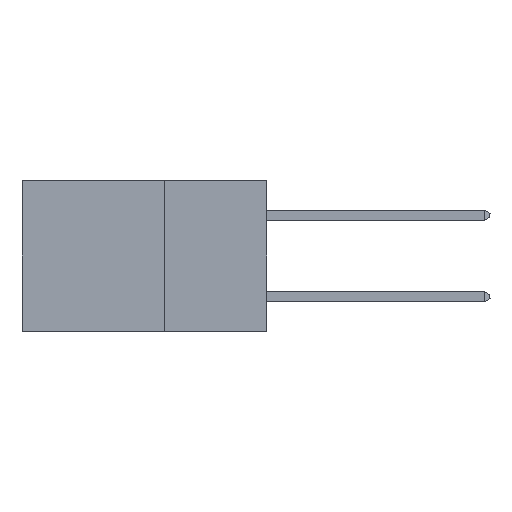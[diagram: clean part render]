
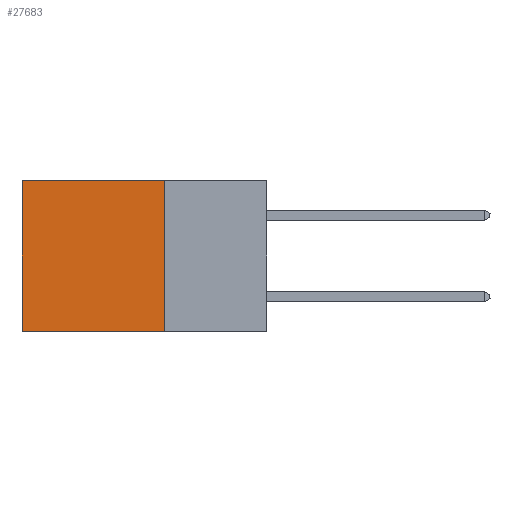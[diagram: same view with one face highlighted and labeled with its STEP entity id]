
A CAD part, left-side view. The second image highlights one B-rep face of the part: STEP entity #27683.
In plain terms, the highlighted planar face has unit normal (-1, 0, 0).
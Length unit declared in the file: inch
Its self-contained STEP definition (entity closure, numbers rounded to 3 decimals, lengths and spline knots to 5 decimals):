
#198 = ORIENTED_EDGE ( 'NONE', *, *, #32950, .F. ) ;
#1918 = CARTESIAN_POINT ( 'NONE',  ( 0.2875, 0.25, 0. ) ) ;
#1966 = EDGE_CURVE ( 'NONE', #16338, #22198, #33736, .T. ) ;
#5202 = AXIS2_PLACEMENT_3D ( 'NONE', #1918, #29483, #35114 ) ;
#5299 = EDGE_LOOP ( 'NONE', ( #31467, #198, #10802, #31281 ) ) ;
#10364 = CARTESIAN_POINT ( 'NONE',  ( 0.2875, 0.25, -0.37 ) ) ;
#10802 = ORIENTED_EDGE ( 'NONE', *, *, #34431, .F. ) ;
#13777 = VERTEX_POINT ( 'NONE', #35957 ) ;
#14352 = CARTESIAN_POINT ( 'NONE',  ( 0.2875, 0.25, 0. ) ) ;
#15483 = VECTOR ( 'NONE', #22196, 39.37008 ) ;
#16338 = VERTEX_POINT ( 'NONE', #34121 ) ;
#17976 = VECTOR ( 'NONE', #29863, 39.37008 ) ;
#19088 = VECTOR ( 'NONE', #32189, 39.37008 ) ;
#19768 = CARTESIAN_POINT ( 'NONE',  ( 0.2875, 0.25, -0.37 ) ) ;
#21308 = VERTEX_POINT ( 'NONE', #19768 ) ;
#21587 = VECTOR ( 'NONE', #33674, 39.37008 ) ;
#22196 = DIRECTION ( 'NONE',  ( 0., 0., -1. ) ) ;
#22198 = VERTEX_POINT ( 'NONE', #22245 ) ;
#22245 = CARTESIAN_POINT ( 'NONE',  ( 0.2875, 0.6, 0. ) ) ;
#22424 = LINE ( 'NONE', #30030, #15483 ) ;
#24116 = PLANE ( 'NONE',  #5202 ) ;
#24154 = EDGE_CURVE ( 'NONE', #22198, #13777, #22424, .T. ) ;
#25229 = LINE ( 'NONE', #10364, #19088 ) ;
#27683 = ADVANCED_FACE ( 'NONE', ( #29589 ), #24116, .F. ) ;
#29025 = LINE ( 'NONE', #14352, #21587 ) ;
#29483 = DIRECTION ( 'NONE',  ( 1., 0., 0. ) ) ;
#29589 = FACE_OUTER_BOUND ( 'NONE', #5299, .T. ) ;
#29863 = DIRECTION ( 'NONE',  ( 0., 1., 0. ) ) ;
#30030 = CARTESIAN_POINT ( 'NONE',  ( 0.2875, 0.6, 0. ) ) ;
#31281 = ORIENTED_EDGE ( 'NONE', *, *, #1966, .T. ) ;
#31467 = ORIENTED_EDGE ( 'NONE', *, *, #24154, .T. ) ;
#32189 = DIRECTION ( 'NONE',  ( 0., 1., 0. ) ) ;
#32950 = EDGE_CURVE ( 'NONE', #21308, #13777, #25229, .T. ) ;
#33674 = DIRECTION ( 'NONE',  ( 0., 0., -1. ) ) ;
#33736 = LINE ( 'NONE', #33966, #17976 ) ;
#33966 = CARTESIAN_POINT ( 'NONE',  ( 0.2875, 0.25, 0. ) ) ;
#34121 = CARTESIAN_POINT ( 'NONE',  ( 0.2875, 0.25, 0. ) ) ;
#34431 = EDGE_CURVE ( 'NONE', #16338, #21308, #29025, .T. ) ;
#35114 = DIRECTION ( 'NONE',  ( 0., 0., -1. ) ) ;
#35957 = CARTESIAN_POINT ( 'NONE',  ( 0.2875, 0.6, -0.37 ) ) ;
